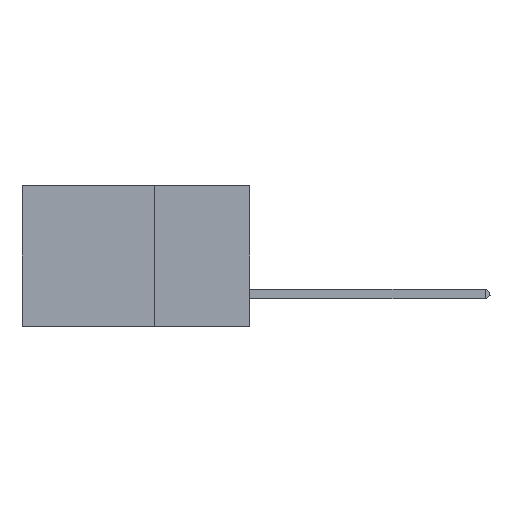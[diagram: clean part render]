
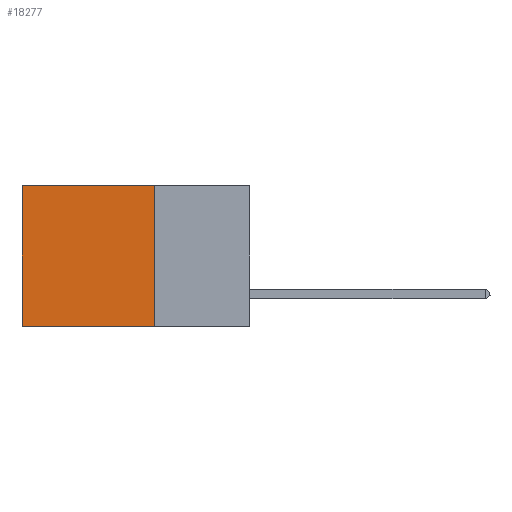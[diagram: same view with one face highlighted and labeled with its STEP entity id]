
A CAD part, left-side view. The second image highlights one B-rep face of the part: STEP entity #18277.
In plain terms, the highlighted planar face has unit normal (-1, 0, 0).
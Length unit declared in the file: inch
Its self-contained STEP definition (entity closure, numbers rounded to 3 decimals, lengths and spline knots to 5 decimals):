
#464 = VECTOR ( 'NONE', #12256, 39.37008 ) ;
#909 = EDGE_CURVE ( 'NONE', #3857, #6283, #18591, .T. ) ;
#1139 = CARTESIAN_POINT ( 'NONE',  ( 0.2875, 0.6, -0.37 ) ) ;
#1140 = EDGE_CURVE ( 'NONE', #8076, #17446, #6298, .T. ) ;
#2084 = DIRECTION ( 'NONE',  ( 0., 0., -1. ) ) ;
#2303 = VECTOR ( 'NONE', #15525, 39.37008 ) ;
#3131 = ORIENTED_EDGE ( 'NONE', *, *, #909, .T. ) ;
#3188 = FACE_OUTER_BOUND ( 'NONE', #10187, .T. ) ;
#3857 = VERTEX_POINT ( 'NONE', #6014 ) ;
#4045 = VECTOR ( 'NONE', #9977, 39.37008 ) ;
#4951 = DIRECTION ( 'NONE',  ( 1., 0., 0. ) ) ;
#5605 = CARTESIAN_POINT ( 'NONE',  ( 0.2875, 0.25, 0. ) ) ;
#5614 = CARTESIAN_POINT ( 'NONE',  ( 0.2875, 0.25, 0. ) ) ;
#6014 = CARTESIAN_POINT ( 'NONE',  ( 0.2875, 0.6, 0. ) ) ;
#6283 = VERTEX_POINT ( 'NONE', #1139 ) ;
#6298 = LINE ( 'NONE', #12413, #2303 ) ;
#7048 = AXIS2_PLACEMENT_3D ( 'NONE', #8048, #4951, #2084 ) ;
#7241 = EDGE_CURVE ( 'NONE', #8076, #3857, #14098, .T. ) ;
#7741 = ORIENTED_EDGE ( 'NONE', *, *, #7241, .T. ) ;
#8048 = CARTESIAN_POINT ( 'NONE',  ( 0.2875, 0.25, 0. ) ) ;
#8076 = VERTEX_POINT ( 'NONE', #5605 ) ;
#9977 = DIRECTION ( 'NONE',  ( 0., 1., 0. ) ) ;
#10187 = EDGE_LOOP ( 'NONE', ( #3131, #17781, #11791, #7741 ) ) ;
#11645 = VECTOR ( 'NONE', #14167, 39.37008 ) ;
#11791 = ORIENTED_EDGE ( 'NONE', *, *, #1140, .F. ) ;
#12256 = DIRECTION ( 'NONE',  ( 0., 0., -1. ) ) ;
#12413 = CARTESIAN_POINT ( 'NONE',  ( 0.2875, 0.25, 0. ) ) ;
#13400 = EDGE_CURVE ( 'NONE', #17446, #6283, #16764, .T. ) ;
#13892 = PLANE ( 'NONE',  #7048 ) ;
#14098 = LINE ( 'NONE', #5614, #4045 ) ;
#14167 = DIRECTION ( 'NONE',  ( 0., 1., 0. ) ) ;
#15525 = DIRECTION ( 'NONE',  ( 0., 0., -1. ) ) ;
#15766 = CARTESIAN_POINT ( 'NONE',  ( 0.2875, 0.25, -0.37 ) ) ;
#16764 = LINE ( 'NONE', #15766, #11645 ) ;
#17446 = VERTEX_POINT ( 'NONE', #18838 ) ;
#17781 = ORIENTED_EDGE ( 'NONE', *, *, #13400, .F. ) ;
#18277 = ADVANCED_FACE ( 'NONE', ( #3188 ), #13892, .F. ) ;
#18472 = CARTESIAN_POINT ( 'NONE',  ( 0.2875, 0.6, 0. ) ) ;
#18591 = LINE ( 'NONE', #18472, #464 ) ;
#18838 = CARTESIAN_POINT ( 'NONE',  ( 0.2875, 0.25, -0.37 ) ) ;
